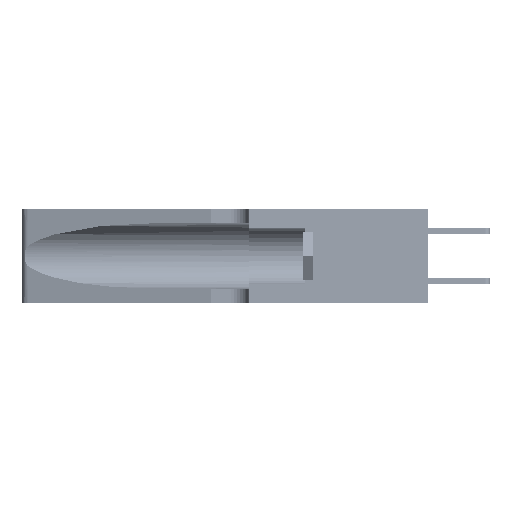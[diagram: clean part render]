
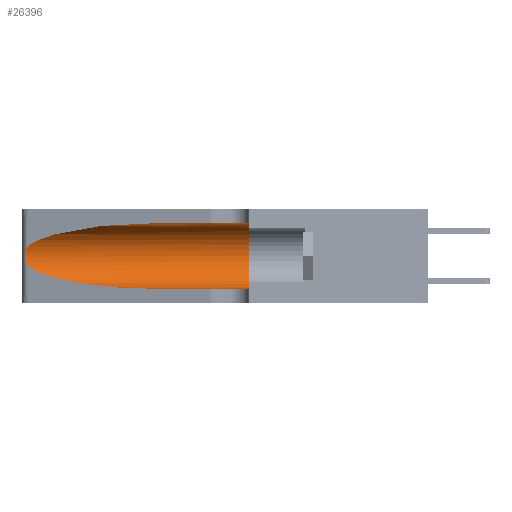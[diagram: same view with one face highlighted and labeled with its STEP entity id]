
A CAD part, left-side view. The second image highlights one B-rep face of the part: STEP entity #26396.
In plain terms, the highlighted cylindrical face has radius 3.308 mm (diameter 6.617 mm), a partial arc.
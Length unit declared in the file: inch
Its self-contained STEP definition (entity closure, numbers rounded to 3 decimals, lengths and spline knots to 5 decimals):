
#1492 = CARTESIAN_POINT ( 'NONE',  ( 0.25856, 1.23593, 0.16098 ) ) ;
#2072 = ORIENTED_EDGE ( 'NONE', *, *, #17666, .F. ) ;
#2118 = ORIENTED_EDGE ( 'NONE', *, *, #15741, .T. ) ;
#2594 = ORIENTED_EDGE ( 'NONE', *, *, #6415, .T. ) ;
#2622 = VECTOR ( 'NONE', #40389, 39.37008 ) ;
#3215 = CARTESIAN_POINT ( 'NONE',  ( 0.1305, 1.61858, 0.31525 ) ) ;
#3224 = VERTEX_POINT ( 'NONE', #40094 ) ;
#4704 = CARTESIAN_POINT ( 'NONE',  ( 0.25555, 1.22993, 0.14849 ) ) ;
#5998 = EDGE_CURVE ( 'NONE', #31741, #8060, #13113, .T. ) ;
#6415 = EDGE_CURVE ( 'NONE', #7602, #8060, #12098, .T. ) ;
#7493 = CARTESIAN_POINT ( 'NONE',  ( 0.1305, 0.35, 0.185 ) ) ;
#7602 = VERTEX_POINT ( 'NONE', #17703 ) ;
#8060 = VERTEX_POINT ( 'NONE', #15790 ) ;
#8065 = CARTESIAN_POINT ( 'NONE',  ( 0.26075, 1.23896, 0.178 ) ) ;
#9287 = CARTESIAN_POINT ( 'NONE',  ( 0.2373, 1.15595, 0.28018 ) ) ;
#9772 = VERTEX_POINT ( 'NONE', #14740 ) ;
#10315 = CARTESIAN_POINT ( 'NONE',  ( 0.1305, 0.72297, 0.05475 ) ) ;
#10528 = ORIENTED_EDGE ( 'NONE', *, *, #38915, .T. ) ;
#10585 = EDGE_LOOP ( 'NONE', ( #27685, #10528, #2118, #2594, #35662, #2072 ) ) ;
#10981 = CARTESIAN_POINT ( 'NONE',  ( 0.25555, 1.22994, 0.2215 ) ) ;
#11583 = DIRECTION ( 'NONE',  ( 0., 0., -1. ) ) ;
#11869 = CARTESIAN_POINT ( 'NONE',  ( 0.1305, 1.61858, 0.185 ) ) ;
#12098 = LINE ( 'NONE', #14773, #2622 ) ;
#13113 = CIRCLE ( 'NONE', #29253, 0.13025 ) ;
#14025 = CARTESIAN_POINT ( 'NONE',  ( 0.25789, 1.23486, 0.15765 ) ) ;
#14740 = CARTESIAN_POINT ( 'NONE',  ( 0.25487, 1.22718, 0.14631 ) ) ;
#14773 = CARTESIAN_POINT ( 'NONE',  ( 0.1305, 1.61858, 0.05475 ) ) ;
#15226 = EDGE_CURVE ( 'NONE', #3224, #22738, #19215, .T. ) ;
#15741 = EDGE_CURVE ( 'NONE', #9772, #7602, #37042, .T. ) ;
#15790 = CARTESIAN_POINT ( 'NONE',  ( 0.1305, 0.35, 0.05475 ) ) ;
#16739 = VECTOR ( 'NONE', #25813, 39.37008 ) ;
#17050 = DIRECTION ( 'NONE',  ( 0., 1., 0. ) ) ;
#17211 = CARTESIAN_POINT ( 'NONE',  ( 0.25639, 1.23186, 0.15144 ) ) ;
#17468 = CARTESIAN_POINT ( 'NONE',  ( 0.25854, 1.2359, 0.20912 ) ) ;
#17666 = EDGE_CURVE ( 'NONE', #3224, #31741, #22660, .T. ) ;
#17703 = CARTESIAN_POINT ( 'NONE',  ( 0.1305, 0.72297, 0.05475 ) ) ;
#19139 = CARTESIAN_POINT ( 'NONE',  ( 0.2373, 1.15595, 0.08982 ) ) ;
#19215 =( BOUNDED_CURVE ( )  B_SPLINE_CURVE ( 3, ( #40428, #27951, #9287, #40691 ),
 .UNSPECIFIED., .F., .F. ) 
 B_SPLINE_CURVE_WITH_KNOTS ( ( 4, 4 ),
 ( 1.5708, 2.84003 ),
 .UNSPECIFIED. ) 
 CURVE ( )  GEOMETRIC_REPRESENTATION_ITEM ( )  RATIONAL_B_SPLINE_CURVE ( ( 1., 0.87, 0.87, 1. ) ) 
 REPRESENTATION_ITEM ( '' )  );
#19679 = FACE_OUTER_BOUND ( 'NONE', #10585, .T. ) ;
#20497 = CARTESIAN_POINT ( 'NONE',  ( 0.26017, 1.23833, 0.17102 ) ) ;
#22272 = B_SPLINE_CURVE_WITH_KNOTS ( 'NONE', 3,
 ( #29937, #10981, #30356, #36473, #17468, #33137, #39503, #8065, #20497, #1492, #14025, #17211, #4704, #39643 ),
 .UNSPECIFIED., .F., .F.,
 ( 4, 2, 2, 2, 2, 2, 4 ),
 ( 0., 0.00027, 0.00053, 0.00107, 0.0016, 0.00187, 0.00214 ),
 .UNSPECIFIED. ) ;
#22660 = LINE ( 'NONE', #3215, #16739 ) ;
#22738 = VERTEX_POINT ( 'NONE', #38004 ) ;
#23609 = AXIS2_PLACEMENT_3D ( 'NONE', #11869, #34150, #11583 ) ;
#25675 = CYLINDRICAL_SURFACE ( 'NONE', #23609, 0.13025 ) ;
#25813 = DIRECTION ( 'NONE',  ( 0., -1., 0. ) ) ;
#26396 = ADVANCED_FACE ( 'NONE', ( #19679 ), #25675, .F. ) ;
#27685 = ORIENTED_EDGE ( 'NONE', *, *, #15226, .T. ) ;
#27951 = CARTESIAN_POINT ( 'NONE',  ( 0.18966, 0.96281, 0.31525 ) ) ;
#28712 = CARTESIAN_POINT ( 'NONE',  ( 0.18966, 0.96281, 0.05475 ) ) ;
#29253 = AXIS2_PLACEMENT_3D ( 'NONE', #7493, #17050, #35909 ) ;
#29937 = CARTESIAN_POINT ( 'NONE',  ( 0.25487, 1.22718, 0.22369 ) ) ;
#30356 = CARTESIAN_POINT ( 'NONE',  ( 0.25639, 1.23184, 0.21858 ) ) ;
#31741 = VERTEX_POINT ( 'NONE', #36605 ) ;
#33137 = CARTESIAN_POINT ( 'NONE',  ( 0.26018, 1.23835, 0.19895 ) ) ;
#34150 = DIRECTION ( 'NONE',  ( 0., -1., 0. ) ) ;
#35662 = ORIENTED_EDGE ( 'NONE', *, *, #5998, .F. ) ;
#35909 = DIRECTION ( 'NONE',  ( 0., 0., 1. ) ) ;
#36473 = CARTESIAN_POINT ( 'NONE',  ( 0.25787, 1.23484, 0.2124 ) ) ;
#36605 = CARTESIAN_POINT ( 'NONE',  ( 0.1305, 0.35, 0.31525 ) ) ;
#37042 =( BOUNDED_CURVE ( )  B_SPLINE_CURVE ( 3, ( #38153, #19139, #28712, #10315 ),
 .UNSPECIFIED., .F., .F. ) 
 B_SPLINE_CURVE_WITH_KNOTS ( ( 4, 4 ),
 ( 3.44316, 4.71239 ),
 .UNSPECIFIED. ) 
 CURVE ( )  GEOMETRIC_REPRESENTATION_ITEM ( )  RATIONAL_B_SPLINE_CURVE ( ( 1., 0.87, 0.87, 1. ) ) 
 REPRESENTATION_ITEM ( '' )  );
#38004 = CARTESIAN_POINT ( 'NONE',  ( 0.25487, 1.22718, 0.22369 ) ) ;
#38153 = CARTESIAN_POINT ( 'NONE',  ( 0.25487, 1.22718, 0.14631 ) ) ;
#38915 = EDGE_CURVE ( 'NONE', #22738, #9772, #22272, .T. ) ;
#39503 = CARTESIAN_POINT ( 'NONE',  ( 0.26075, 1.23896, 0.19203 ) ) ;
#39643 = CARTESIAN_POINT ( 'NONE',  ( 0.25487, 1.22718, 0.14631 ) ) ;
#40094 = CARTESIAN_POINT ( 'NONE',  ( 0.1305, 0.72297, 0.31525 ) ) ;
#40389 = DIRECTION ( 'NONE',  ( 0., -1., 0. ) ) ;
#40428 = CARTESIAN_POINT ( 'NONE',  ( 0.1305, 0.72297, 0.31525 ) ) ;
#40691 = CARTESIAN_POINT ( 'NONE',  ( 0.25487, 1.22718, 0.22369 ) ) ;
